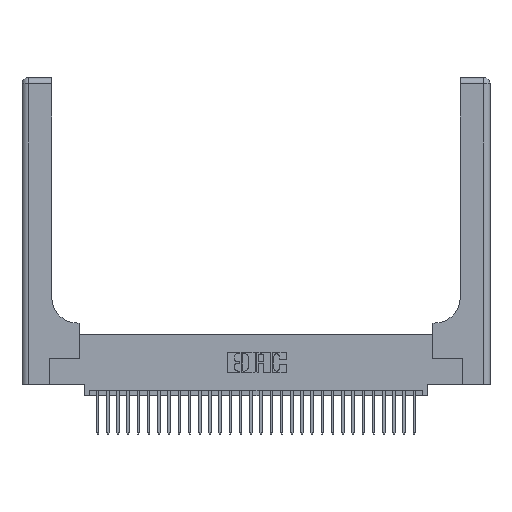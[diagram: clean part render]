
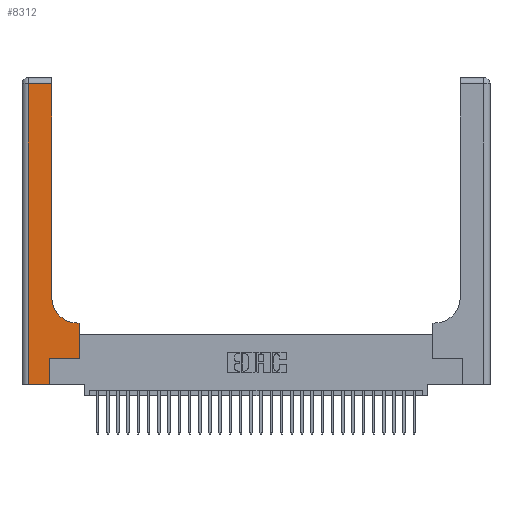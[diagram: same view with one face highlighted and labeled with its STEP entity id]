
A CAD part, top view. The second image highlights one B-rep face of the part: STEP entity #8312.
In plain terms, the highlighted planar face has unit normal (0, 0, 1).
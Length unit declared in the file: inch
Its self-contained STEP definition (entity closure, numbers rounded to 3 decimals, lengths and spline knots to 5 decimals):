
#396 = CARTESIAN_POINT ( 'NONE',  ( 0.2915, 0.6, 0.37 ) ) ;
#679 = DIRECTION ( 'NONE',  ( 1., 0., 0. ) ) ;
#904 = DIRECTION ( 'NONE',  ( 0., 0., -1. ) ) ;
#1501 = VERTEX_POINT ( 'NONE', #13754 ) ;
#1931 = CARTESIAN_POINT ( 'NONE',  ( 0.5585, 0.25, 0.37 ) ) ;
#1951 = CARTESIAN_POINT ( 'NONE',  ( 0.269, 0., 0.37 ) ) ;
#2000 = EDGE_CURVE ( 'NONE', #8528, #16359, #14809, .T. ) ;
#2002 = LINE ( 'NONE', #12233, #2354 ) ;
#2068 = CARTESIAN_POINT ( 'NONE',  ( 0., 3., 0.37 ) ) ;
#2354 = VECTOR ( 'NONE', #17087, 39.37008 ) ;
#2531 = CARTESIAN_POINT ( 'NONE',  ( 0.5585, 0.6, 0.37 ) ) ;
#2853 = VECTOR ( 'NONE', #18438, 39.37008 ) ;
#3397 = CARTESIAN_POINT ( 'NONE',  ( 0.06, 3., 0.37 ) ) ;
#4098 = AXIS2_PLACEMENT_3D ( 'NONE', #2068, #24299, #24185 ) ;
#5019 = CARTESIAN_POINT ( 'NONE',  ( 0.2915, 3., 0.37 ) ) ;
#5066 = AXIS2_PLACEMENT_3D ( 'NONE', #25074, #904, #679 ) ;
#5159 = EDGE_CURVE ( 'NONE', #9118, #1501, #17876, .T. ) ;
#5640 = CIRCLE ( 'NONE', #5066, 0.25 ) ;
#6251 = DIRECTION ( 'NONE',  ( 1., 0., 0. ) ) ;
#6738 = VECTOR ( 'NONE', #11360, 39.37008 ) ;
#7207 = ORIENTED_EDGE ( 'NONE', *, *, #5159, .T. ) ;
#8312 = ADVANCED_FACE ( 'NONE', ( #17345 ), #16765, .F. ) ;
#8474 = LINE ( 'NONE', #23650, #23478 ) ;
#8528 = VERTEX_POINT ( 'NONE', #15565 ) ;
#9112 = LINE ( 'NONE', #25842, #31408 ) ;
#9118 = VERTEX_POINT ( 'NONE', #1951 ) ;
#9357 = LINE ( 'NONE', #5019, #22075 ) ;
#10229 = CARTESIAN_POINT ( 'NONE',  ( 0.5415, 0.6, 0.37 ) ) ;
#11159 = EDGE_CURVE ( 'NONE', #25518, #29570, #12536, .T. ) ;
#11360 = DIRECTION ( 'NONE',  ( 0., 1., 0. ) ) ;
#11461 = CARTESIAN_POINT ( 'NONE',  ( 0.269, 0., 0.37 ) ) ;
#11776 = ORIENTED_EDGE ( 'NONE', *, *, #2000, .T. ) ;
#12233 = CARTESIAN_POINT ( 'NONE',  ( 0., 2.94, 0.37 ) ) ;
#12536 = LINE ( 'NONE', #396, #21751 ) ;
#12660 = LINE ( 'NONE', #16945, #18037 ) ;
#13405 = EDGE_CURVE ( 'NONE', #17614, #8528, #2002, .T. ) ;
#13754 = CARTESIAN_POINT ( 'NONE',  ( 0.269, 0.25, 0.37 ) ) ;
#14400 = CARTESIAN_POINT ( 'NONE',  ( 0.2915, 0.85, 0.37 ) ) ;
#14809 = LINE ( 'NONE', #3397, #2853 ) ;
#15325 = ORIENTED_EDGE ( 'NONE', *, *, #21811, .T. ) ;
#15565 = CARTESIAN_POINT ( 'NONE',  ( 0.06, 2.94, 0.37 ) ) ;
#15740 = ORIENTED_EDGE ( 'NONE', *, *, #22143, .T. ) ;
#16173 = VERTEX_POINT ( 'NONE', #14400 ) ;
#16359 = VERTEX_POINT ( 'NONE', #17490 ) ;
#16765 = PLANE ( 'NONE',  #4098 ) ;
#16945 = CARTESIAN_POINT ( 'NONE',  ( 0.269, 0.25, 0.37 ) ) ;
#17087 = DIRECTION ( 'NONE',  ( -1., 0., 0. ) ) ;
#17345 = FACE_OUTER_BOUND ( 'NONE', #22720, .T. ) ;
#17490 = CARTESIAN_POINT ( 'NONE',  ( 0.06, 0., 0.37 ) ) ;
#17614 = VERTEX_POINT ( 'NONE', #25428 ) ;
#17876 = LINE ( 'NONE', #11461, #6738 ) ;
#17993 = DIRECTION ( 'NONE',  ( 0., 1., 0. ) ) ;
#18037 = VECTOR ( 'NONE', #24151, 39.37008 ) ;
#18438 = DIRECTION ( 'NONE',  ( 0., -1., 0. ) ) ;
#18851 = ORIENTED_EDGE ( 'NONE', *, *, #19219, .T. ) ;
#18924 = ORIENTED_EDGE ( 'NONE', *, *, #11159, .T. ) ;
#19219 = EDGE_CURVE ( 'NONE', #16359, #9118, #8474, .T. ) ;
#19988 = EDGE_CURVE ( 'NONE', #1501, #30777, #12660, .T. ) ;
#21751 = VECTOR ( 'NONE', #24779, 39.37008 ) ;
#21811 = EDGE_CURVE ( 'NONE', #30777, #25518, #9112, .T. ) ;
#22018 = ORIENTED_EDGE ( 'NONE', *, *, #19988, .T. ) ;
#22075 = VECTOR ( 'NONE', #17993, 39.37008 ) ;
#22143 = EDGE_CURVE ( 'NONE', #29570, #16173, #5640, .T. ) ;
#22720 = EDGE_LOOP ( 'NONE', ( #27238, #28230, #11776, #18851, #7207, #22018, #15325, #18924, #15740 ) ) ;
#23478 = VECTOR ( 'NONE', #6251, 39.37008 ) ;
#23650 = CARTESIAN_POINT ( 'NONE',  ( 0., 0., 0.37 ) ) ;
#24151 = DIRECTION ( 'NONE',  ( 1., 0., 0. ) ) ;
#24185 = DIRECTION ( 'NONE',  ( -1., 0., 0. ) ) ;
#24299 = DIRECTION ( 'NONE',  ( 0., 0., -1. ) ) ;
#24779 = DIRECTION ( 'NONE',  ( -1., 0., 0. ) ) ;
#25074 = CARTESIAN_POINT ( 'NONE',  ( 0.5415, 0.85, 0.37 ) ) ;
#25428 = CARTESIAN_POINT ( 'NONE',  ( 0.2915, 2.94, 0.37 ) ) ;
#25518 = VERTEX_POINT ( 'NONE', #2531 ) ;
#25569 = EDGE_CURVE ( 'NONE', #16173, #17614, #9357, .T. ) ;
#25842 = CARTESIAN_POINT ( 'NONE',  ( 0.5585, 0.25, 0.37 ) ) ;
#27238 = ORIENTED_EDGE ( 'NONE', *, *, #25569, .T. ) ;
#28230 = ORIENTED_EDGE ( 'NONE', *, *, #13405, .T. ) ;
#29570 = VERTEX_POINT ( 'NONE', #10229 ) ;
#30777 = VERTEX_POINT ( 'NONE', #1931 ) ;
#31087 = DIRECTION ( 'NONE',  ( 0., 1., 0. ) ) ;
#31408 = VECTOR ( 'NONE', #31087, 39.37008 ) ;
